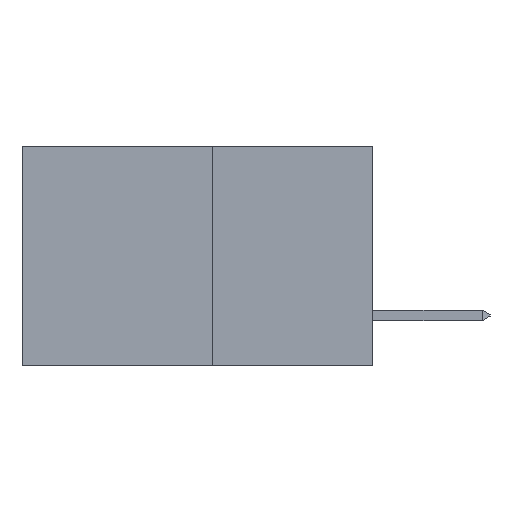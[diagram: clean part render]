
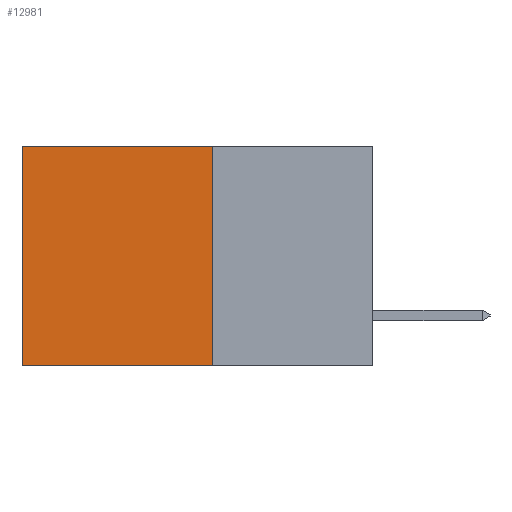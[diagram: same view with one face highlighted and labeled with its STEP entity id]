
A CAD part, left-side view. The second image highlights one B-rep face of the part: STEP entity #12981.
In plain terms, the highlighted planar face has unit normal (-1, 0, 0).
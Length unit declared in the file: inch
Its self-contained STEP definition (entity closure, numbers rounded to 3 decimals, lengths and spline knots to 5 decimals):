
#208 = DIRECTION ( 'NONE',  ( 0., 0., -1. ) ) ;
#1356 = LINE ( 'NONE', #8437, #5831 ) ;
#1539 = EDGE_CURVE ( 'NONE', #11215, #5776, #19808, .T. ) ;
#2092 = ORIENTED_EDGE ( 'NONE', *, *, #1539, .T. ) ;
#3668 = DIRECTION ( 'NONE',  ( 0., 1., 0. ) ) ;
#4380 = CARTESIAN_POINT ( 'NONE',  ( 0.277, 0.59, 0. ) ) ;
#5776 = VERTEX_POINT ( 'NONE', #17315 ) ;
#5831 = VECTOR ( 'NONE', #19770, 39.37008 ) ;
#6735 = LINE ( 'NONE', #9317, #21251 ) ;
#7272 = CARTESIAN_POINT ( 'NONE',  ( 0.277, 0.27, 0. ) ) ;
#7744 = EDGE_LOOP ( 'NONE', ( #2092, #7771, #19540, #19768 ) ) ;
#7771 = ORIENTED_EDGE ( 'NONE', *, *, #10267, .F. ) ;
#7916 = DIRECTION ( 'NONE',  ( 0., 0., -1. ) ) ;
#8437 = CARTESIAN_POINT ( 'NONE',  ( 0.277, 0.27, -0.37 ) ) ;
#9317 = CARTESIAN_POINT ( 'NONE',  ( 0.277, 0.27, -0.37 ) ) ;
#9774 = PLANE ( 'NONE',  #18093 ) ;
#10267 = EDGE_CURVE ( 'NONE', #13888, #5776, #6735, .T. ) ;
#11215 = VERTEX_POINT ( 'NONE', #4380 ) ;
#11370 = CARTESIAN_POINT ( 'NONE',  ( 0.277, 0.27, 0. ) ) ;
#11705 = DIRECTION ( 'NONE',  ( 1., 0., 0. ) ) ;
#12981 = ADVANCED_FACE ( 'NONE', ( #20854 ), #9774, .F. ) ;
#13888 = VERTEX_POINT ( 'NONE', #20505 ) ;
#14854 = VECTOR ( 'NONE', #7916, 39.37008 ) ;
#16895 = DIRECTION ( 'NONE',  ( 0., 1., 0. ) ) ;
#17066 = EDGE_CURVE ( 'NONE', #23415, #11215, #19603, .T. ) ;
#17315 = CARTESIAN_POINT ( 'NONE',  ( 0.277, 0.59, -0.37 ) ) ;
#18093 = AXIS2_PLACEMENT_3D ( 'NONE', #22900, #11705, #208 ) ;
#18953 = CARTESIAN_POINT ( 'NONE',  ( 0.277, 0.59, -0.37 ) ) ;
#19098 = EDGE_CURVE ( 'NONE', #23415, #13888, #1356, .T. ) ;
#19540 = ORIENTED_EDGE ( 'NONE', *, *, #19098, .F. ) ;
#19603 = LINE ( 'NONE', #7272, #23904 ) ;
#19768 = ORIENTED_EDGE ( 'NONE', *, *, #17066, .T. ) ;
#19770 = DIRECTION ( 'NONE',  ( 0., 0., -1. ) ) ;
#19808 = LINE ( 'NONE', #18953, #14854 ) ;
#20505 = CARTESIAN_POINT ( 'NONE',  ( 0.277, 0.27, -0.37 ) ) ;
#20854 = FACE_OUTER_BOUND ( 'NONE', #7744, .T. ) ;
#21251 = VECTOR ( 'NONE', #3668, 39.37008 ) ;
#22900 = CARTESIAN_POINT ( 'NONE',  ( 0.277, 0.27, -0.37 ) ) ;
#23415 = VERTEX_POINT ( 'NONE', #11370 ) ;
#23904 = VECTOR ( 'NONE', #16895, 39.37008 ) ;
